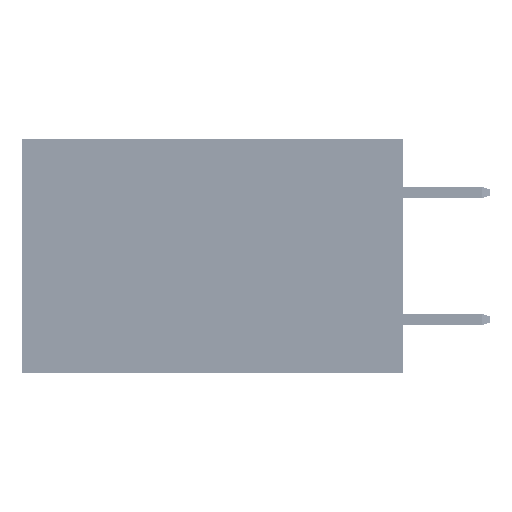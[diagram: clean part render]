
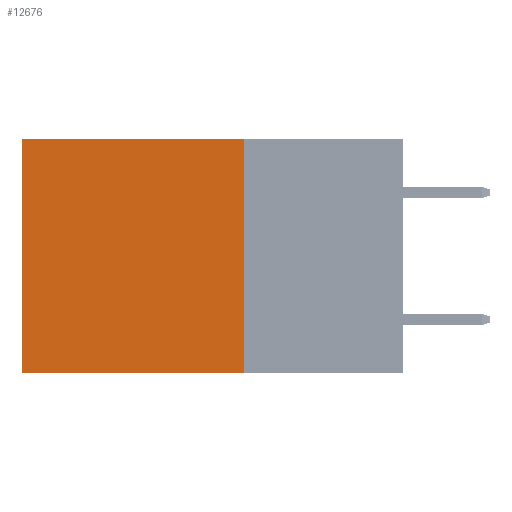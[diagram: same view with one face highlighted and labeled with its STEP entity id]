
A CAD part, left-side view. The second image highlights one B-rep face of the part: STEP entity #12676.
In plain terms, the highlighted planar face has unit normal (-1, 0, 0).
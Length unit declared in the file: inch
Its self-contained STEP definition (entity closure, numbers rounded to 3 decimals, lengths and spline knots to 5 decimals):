
#1453 = DIRECTION ( 'NONE',  ( 0., 1., 0. ) ) ;
#4245 = ORIENTED_EDGE ( 'NONE', *, *, #39378, .T. ) ;
#4402 = FACE_OUTER_BOUND ( 'NONE', #47811, .T. ) ;
#4650 = VECTOR ( 'NONE', #9892, 39.37008 ) ;
#5576 = VECTOR ( 'NONE', #1453, 39.37008 ) ;
#9652 = CARTESIAN_POINT ( 'NONE',  ( 0.2875, 0.25, 0. ) ) ;
#9892 = DIRECTION ( 'NONE',  ( 0., 0., -1. ) ) ;
#9912 = LINE ( 'NONE', #9652, #5576 ) ;
#10409 = CARTESIAN_POINT ( 'NONE',  ( 0.2875, 0.6, 0. ) ) ;
#12640 = ORIENTED_EDGE ( 'NONE', *, *, #50202, .F. ) ;
#12676 = ADVANCED_FACE ( 'NONE', ( #4402 ), #16157, .F. ) ;
#14251 = CARTESIAN_POINT ( 'NONE',  ( 0.2875, 0.25, -0.37 ) ) ;
#16157 = PLANE ( 'NONE',  #32702 ) ;
#16530 = CARTESIAN_POINT ( 'NONE',  ( 0.2875, 0.6, -0.37 ) ) ;
#17777 = CARTESIAN_POINT ( 'NONE',  ( 0.2875, 0.6, 0. ) ) ;
#17863 = ORIENTED_EDGE ( 'NONE', *, *, #27407, .T. ) ;
#21980 = VERTEX_POINT ( 'NONE', #16530 ) ;
#27407 = EDGE_CURVE ( 'NONE', #40035, #48218, #9912, .T. ) ;
#30619 = LINE ( 'NONE', #39279, #46197 ) ;
#31411 = DIRECTION ( 'NONE',  ( 0., 1., 0. ) ) ;
#32702 = AXIS2_PLACEMENT_3D ( 'NONE', #35331, #35079, #47350 ) ;
#33898 = LINE ( 'NONE', #17777, #4650 ) ;
#34238 = LINE ( 'NONE', #35236, #46018 ) ;
#35079 = DIRECTION ( 'NONE',  ( 1., 0., 0. ) ) ;
#35236 = CARTESIAN_POINT ( 'NONE',  ( 0.2875, 0.25, -0.37 ) ) ;
#35331 = CARTESIAN_POINT ( 'NONE',  ( 0.2875, 0.25, 0. ) ) ;
#37695 = ORIENTED_EDGE ( 'NONE', *, *, #37739, .F. ) ;
#37739 = EDGE_CURVE ( 'NONE', #40035, #44838, #30619, .T. ) ;
#39279 = CARTESIAN_POINT ( 'NONE',  ( 0.2875, 0.25, 0. ) ) ;
#39378 = EDGE_CURVE ( 'NONE', #48218, #21980, #33898, .T. ) ;
#40035 = VERTEX_POINT ( 'NONE', #40194 ) ;
#40194 = CARTESIAN_POINT ( 'NONE',  ( 0.2875, 0.25, 0. ) ) ;
#44838 = VERTEX_POINT ( 'NONE', #14251 ) ;
#46018 = VECTOR ( 'NONE', #31411, 39.37008 ) ;
#46197 = VECTOR ( 'NONE', #46209, 39.37008 ) ;
#46209 = DIRECTION ( 'NONE',  ( 0., 0., -1. ) ) ;
#47350 = DIRECTION ( 'NONE',  ( 0., 0., -1. ) ) ;
#47811 = EDGE_LOOP ( 'NONE', ( #4245, #12640, #37695, #17863 ) ) ;
#48218 = VERTEX_POINT ( 'NONE', #10409 ) ;
#50202 = EDGE_CURVE ( 'NONE', #44838, #21980, #34238, .T. ) ;
